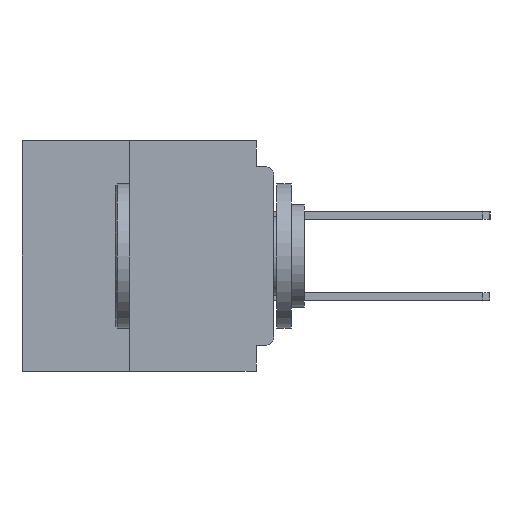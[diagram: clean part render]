
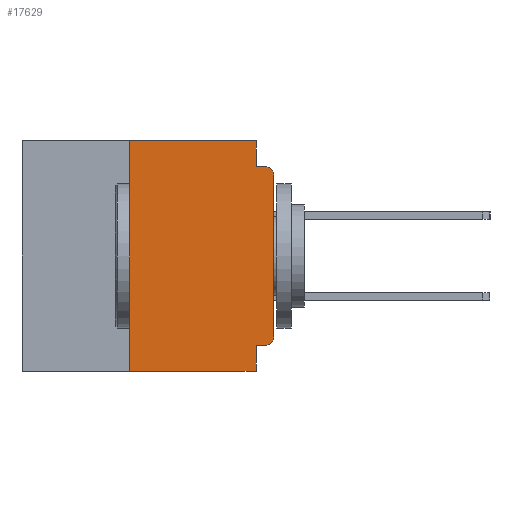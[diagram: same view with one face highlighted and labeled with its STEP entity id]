
A CAD part, left-side view. The second image highlights one B-rep face of the part: STEP entity #17629.
In plain terms, the highlighted planar face has unit normal (-1, 0, 0).
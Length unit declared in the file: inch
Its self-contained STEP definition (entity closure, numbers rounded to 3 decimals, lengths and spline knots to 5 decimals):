
#208 = VERTEX_POINT ( 'NONE', #68515 ) ;
#440 = CARTESIAN_POINT ( 'NONE',  ( 0., 0.031, -0.4 ) ) ;
#1529 = VECTOR ( 'NONE', #64419, 39.37008 ) ;
#3823 = DIRECTION ( 'NONE',  ( 0., 0., -1. ) ) ;
#5728 = ORIENTED_EDGE ( 'NONE', *, *, #20347, .T. ) ;
#6695 = CIRCLE ( 'NONE', #35239, 0.015 ) ;
#7899 = LINE ( 'NONE', #61305, #57935 ) ;
#7956 = CARTESIAN_POINT ( 'NONE',  ( 0., 0.015, -0.34 ) ) ;
#8360 = EDGE_CURVE ( 'NONE', #63898, #54771, #12731, .T. ) ;
#8417 = DIRECTION ( 'NONE',  ( 0., -1., 0. ) ) ;
#8972 = EDGE_CURVE ( 'NONE', #46076, #13647, #27743, .T. ) ;
#10334 = CARTESIAN_POINT ( 'NONE',  ( 0., 0.031, 0. ) ) ;
#12119 = VECTOR ( 'NONE', #19713, 39.37008 ) ;
#12731 = LINE ( 'NONE', #33490, #39432 ) ;
#13332 = DIRECTION ( 'NONE',  ( 0., 0., -1. ) ) ;
#13647 = VERTEX_POINT ( 'NONE', #26993 ) ;
#13688 = EDGE_CURVE ( 'NONE', #13647, #37699, #44182, .T. ) ;
#13802 = VECTOR ( 'NONE', #19830, 39.37008 ) ;
#16080 = EDGE_CURVE ( 'NONE', #54771, #19245, #42198, .T. ) ;
#16833 = CARTESIAN_POINT ( 'NONE',  ( 0., 0.437, 0. ) ) ;
#17291 = EDGE_CURVE ( 'NONE', #22222, #28923, #64504, .T. ) ;
#17629 = ADVANCED_FACE ( 'NONE', ( #25330 ), #27602, .F. ) ;
#18473 = ORIENTED_EDGE ( 'NONE', *, *, #16080, .F. ) ;
#19245 = VERTEX_POINT ( 'NONE', #10334 ) ;
#19602 = CARTESIAN_POINT ( 'NONE',  ( 0., 0.437, 0. ) ) ;
#19713 = DIRECTION ( 'NONE',  ( 0., -1., 0. ) ) ;
#19830 = DIRECTION ( 'NONE',  ( 0., -1., 0. ) ) ;
#20347 = EDGE_CURVE ( 'NONE', #41505, #28923, #28250, .T. ) ;
#22222 = VERTEX_POINT ( 'NONE', #27817 ) ;
#24365 = ORIENTED_EDGE ( 'NONE', *, *, #24489, .T. ) ;
#24489 = EDGE_CURVE ( 'NONE', #46076, #208, #6695, .T. ) ;
#25330 = FACE_OUTER_BOUND ( 'NONE', #41332, .T. ) ;
#25662 = CARTESIAN_POINT ( 'NONE',  ( 0., 0.031, 0. ) ) ;
#26993 = CARTESIAN_POINT ( 'NONE',  ( 0., 0.031, -0.355 ) ) ;
#27362 = ORIENTED_EDGE ( 'NONE', *, *, #13688, .F. ) ;
#27530 = AXIS2_PLACEMENT_3D ( 'NONE', #67691, #35875, #3823 ) ;
#27602 = PLANE ( 'NONE',  #65362 ) ;
#27743 = LINE ( 'NONE', #29008, #29412 ) ;
#27817 = CARTESIAN_POINT ( 'NONE',  ( 0., 0.031, -0.045 ) ) ;
#28250 = CIRCLE ( 'NONE', #27530, 0.015 ) ;
#28442 = CARTESIAN_POINT ( 'NONE',  ( 0., 0.25, -0.4 ) ) ;
#28923 = VERTEX_POINT ( 'NONE', #62938 ) ;
#29008 = CARTESIAN_POINT ( 'NONE',  ( 0., 0., -0.355 ) ) ;
#29412 = VECTOR ( 'NONE', #50119, 39.37008 ) ;
#31445 = ORIENTED_EDGE ( 'NONE', *, *, #37991, .F. ) ;
#32950 = DIRECTION ( 'NONE',  ( 0., 0., -1. ) ) ;
#33490 = CARTESIAN_POINT ( 'NONE',  ( 0., 0.25, -0.4 ) ) ;
#34821 = DIRECTION ( 'NONE',  ( 0., 0., 1. ) ) ;
#35075 = CARTESIAN_POINT ( 'NONE',  ( 0., 0., -0.045 ) ) ;
#35239 = AXIS2_PLACEMENT_3D ( 'NONE', #7956, #45269, #13332 ) ;
#35334 = ORIENTED_EDGE ( 'NONE', *, *, #64755, .T. ) ;
#35875 = DIRECTION ( 'NONE',  ( -1., 0., 0. ) ) ;
#36198 = VECTOR ( 'NONE', #8417, 39.37008 ) ;
#36998 = CARTESIAN_POINT ( 'NONE',  ( 0., 0., -0.06 ) ) ;
#37699 = VERTEX_POINT ( 'NONE', #60533 ) ;
#37991 = EDGE_CURVE ( 'NONE', #19245, #22222, #45742, .T. ) ;
#38304 = CARTESIAN_POINT ( 'NONE',  ( 0., 0.25, 0. ) ) ;
#39432 = VECTOR ( 'NONE', #43936, 39.37008 ) ;
#39832 = EDGE_CURVE ( 'NONE', #63898, #37699, #43845, .T. ) ;
#41332 = EDGE_LOOP ( 'NONE', ( #35334, #5728, #65112, #31445, #18473, #42322, #49749, #27362, #52176, #24365 ) ) ;
#41505 = VERTEX_POINT ( 'NONE', #36998 ) ;
#42198 = LINE ( 'NONE', #19602, #13802 ) ;
#42322 = ORIENTED_EDGE ( 'NONE', *, *, #8360, .F. ) ;
#43845 = LINE ( 'NONE', #56926, #12119 ) ;
#43936 = DIRECTION ( 'NONE',  ( 0., 0., 1. ) ) ;
#44182 = LINE ( 'NONE', #440, #1529 ) ;
#45269 = DIRECTION ( 'NONE',  ( -1., 0., 0. ) ) ;
#45742 = LINE ( 'NONE', #25662, #69018 ) ;
#46076 = VERTEX_POINT ( 'NONE', #63393 ) ;
#49749 = ORIENTED_EDGE ( 'NONE', *, *, #39832, .T. ) ;
#50119 = DIRECTION ( 'NONE',  ( 0., 1., 0. ) ) ;
#52176 = ORIENTED_EDGE ( 'NONE', *, *, #8972, .F. ) ;
#54771 = VERTEX_POINT ( 'NONE', #38304 ) ;
#56926 = CARTESIAN_POINT ( 'NONE',  ( 0., 0.437, -0.4 ) ) ;
#57935 = VECTOR ( 'NONE', #34821, 39.37008 ) ;
#60533 = CARTESIAN_POINT ( 'NONE',  ( 0., 0.031, -0.4 ) ) ;
#61305 = CARTESIAN_POINT ( 'NONE',  ( 0., 0., 0. ) ) ;
#62938 = CARTESIAN_POINT ( 'NONE',  ( 0., 0.015, -0.045 ) ) ;
#63393 = CARTESIAN_POINT ( 'NONE',  ( 0., 0.015, -0.355 ) ) ;
#63898 = VERTEX_POINT ( 'NONE', #28442 ) ;
#64419 = DIRECTION ( 'NONE',  ( 0., 0., -1. ) ) ;
#64504 = LINE ( 'NONE', #35075, #36198 ) ;
#64755 = EDGE_CURVE ( 'NONE', #208, #41505, #7899, .T. ) ;
#64791 = DIRECTION ( 'NONE',  ( 1., 0., 0. ) ) ;
#65112 = ORIENTED_EDGE ( 'NONE', *, *, #17291, .F. ) ;
#65362 = AXIS2_PLACEMENT_3D ( 'NONE', #16833, #64791, #32950 ) ;
#67691 = CARTESIAN_POINT ( 'NONE',  ( 0., 0.015, -0.06 ) ) ;
#68162 = DIRECTION ( 'NONE',  ( 0., 0., -1. ) ) ;
#68515 = CARTESIAN_POINT ( 'NONE',  ( 0., 0., -0.34 ) ) ;
#69018 = VECTOR ( 'NONE', #68162, 39.37008 ) ;
